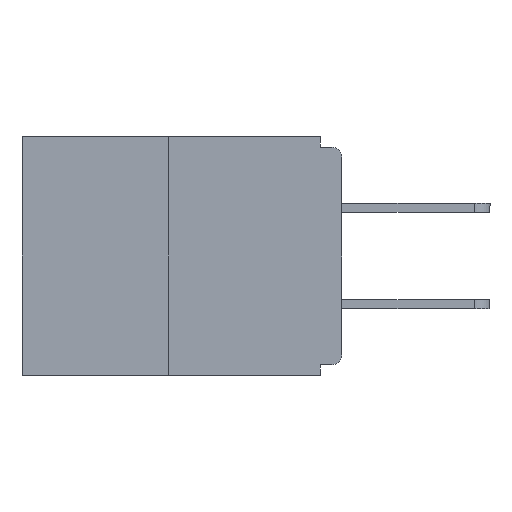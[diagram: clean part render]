
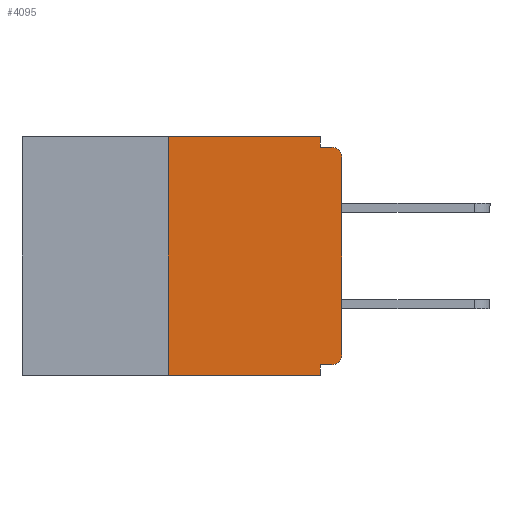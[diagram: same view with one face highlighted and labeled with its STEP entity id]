
A CAD part, left-side view. The second image highlights one B-rep face of the part: STEP entity #4095.
In plain terms, the highlighted planar face has unit normal (-1, 0, 0).
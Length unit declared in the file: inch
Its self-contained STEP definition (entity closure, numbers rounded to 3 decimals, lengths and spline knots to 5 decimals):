
#136 = EDGE_CURVE ( 'NONE', #3939, #10348, #20464, .T. ) ;
#175 = VECTOR ( 'NONE', #2229, 39.37008 ) ;
#220 = CARTESIAN_POINT ( 'NONE',  ( 0., 0.46, 0. ) ) ;
#252 = ORIENTED_EDGE ( 'NONE', *, *, #10432, .F. ) ;
#340 = CARTESIAN_POINT ( 'NONE',  ( 0., 0., -0.03 ) ) ;
#493 = LINE ( 'NONE', #2127, #12126 ) ;
#1427 = VERTEX_POINT ( 'NONE', #12064 ) ;
#2127 = CARTESIAN_POINT ( 'NONE',  ( 0., 0.46, -0.343 ) ) ;
#2229 = DIRECTION ( 'NONE',  ( 0., -1., 0. ) ) ;
#2239 = DIRECTION ( 'NONE',  ( 0., 0., -1. ) ) ;
#2779 = LINE ( 'NONE', #7794, #8220 ) ;
#2801 = CARTESIAN_POINT ( 'NONE',  ( 0., 0.015, -0.015 ) ) ;
#2879 = ORIENTED_EDGE ( 'NONE', *, *, #3324, .F. ) ;
#3036 = EDGE_CURVE ( 'NONE', #13021, #10348, #493, .T. ) ;
#3054 = ORIENTED_EDGE ( 'NONE', *, *, #16053, .F. ) ;
#3324 = EDGE_CURVE ( 'NONE', #13021, #15817, #4747, .T. ) ;
#3610 = CARTESIAN_POINT ( 'NONE',  ( 0., 0.015, -0.328 ) ) ;
#3939 = VERTEX_POINT ( 'NONE', #9247 ) ;
#4095 = ADVANCED_FACE ( 'NONE', ( #6446 ), #19255, .F. ) ;
#4668 = CARTESIAN_POINT ( 'NONE',  ( 0., 0., -0.328 ) ) ;
#4747 = LINE ( 'NONE', #15003, #13897 ) ;
#4929 = CARTESIAN_POINT ( 'NONE',  ( 0., 0.031, 0. ) ) ;
#5041 = CIRCLE ( 'NONE', #9271, 0.015 ) ;
#5063 = LINE ( 'NONE', #4668, #12690 ) ;
#5141 = DIRECTION ( 'NONE',  ( 0., -1., 0. ) ) ;
#5260 = VERTEX_POINT ( 'NONE', #340 ) ;
#5685 = LINE ( 'NONE', #8404, #175 ) ;
#5875 = ORIENTED_EDGE ( 'NONE', *, *, #16326, .T. ) ;
#6446 = FACE_OUTER_BOUND ( 'NONE', #13873, .T. ) ;
#6505 = DIRECTION ( 'NONE',  ( 1., 0., 0. ) ) ;
#6519 = DIRECTION ( 'NONE',  ( 0., 0., -1. ) ) ;
#6920 = ORIENTED_EDGE ( 'NONE', *, *, #15191, .F. ) ;
#7124 = ORIENTED_EDGE ( 'NONE', *, *, #12828, .F. ) ;
#7405 = CARTESIAN_POINT ( 'NONE',  ( 0., 0.46, 0. ) ) ;
#7550 = CARTESIAN_POINT ( 'NONE',  ( 0., 0.031, -0.015 ) ) ;
#7794 = CARTESIAN_POINT ( 'NONE',  ( 0., 0., 0. ) ) ;
#8066 = VERTEX_POINT ( 'NONE', #2801 ) ;
#8220 = VECTOR ( 'NONE', #15786, 39.37008 ) ;
#8404 = CARTESIAN_POINT ( 'NONE',  ( 0., 0., -0.015 ) ) ;
#8545 = VECTOR ( 'NONE', #20500, 39.37008 ) ;
#8614 = DIRECTION ( 'NONE',  ( -1., 0., 0. ) ) ;
#8753 = LINE ( 'NONE', #4929, #11954 ) ;
#8851 = CIRCLE ( 'NONE', #18661, 0.015 ) ;
#9132 = VERTEX_POINT ( 'NONE', #15244 ) ;
#9247 = CARTESIAN_POINT ( 'NONE',  ( 0., 0.031, -0.328 ) ) ;
#9271 = AXIS2_PLACEMENT_3D ( 'NONE', #16479, #8614, #2239 ) ;
#9798 = VERTEX_POINT ( 'NONE', #7550 ) ;
#9909 = DIRECTION ( 'NONE',  ( 0., 0., -1. ) ) ;
#10045 = DIRECTION ( 'NONE',  ( -1., 0., 0. ) ) ;
#10348 = VERTEX_POINT ( 'NONE', #18859 ) ;
#10432 = EDGE_CURVE ( 'NONE', #9132, #9798, #8753, .T. ) ;
#10541 = LINE ( 'NONE', #7405, #11522 ) ;
#11482 = CARTESIAN_POINT ( 'NONE',  ( 0., 0.015, -0.03 ) ) ;
#11522 = VECTOR ( 'NONE', #13494, 39.37008 ) ;
#11954 = VECTOR ( 'NONE', #6519, 39.37008 ) ;
#12064 = CARTESIAN_POINT ( 'NONE',  ( 0., 0., -0.313 ) ) ;
#12126 = VECTOR ( 'NONE', #5141, 39.37008 ) ;
#12532 = DIRECTION ( 'NONE',  ( 0., 1., 0. ) ) ;
#12570 = CARTESIAN_POINT ( 'NONE',  ( 0., 0.031, -0.343 ) ) ;
#12571 = ORIENTED_EDGE ( 'NONE', *, *, #3036, .T. ) ;
#12690 = VECTOR ( 'NONE', #12532, 39.37008 ) ;
#12828 = EDGE_CURVE ( 'NONE', #9798, #8066, #5685, .T. ) ;
#13021 = VERTEX_POINT ( 'NONE', #13996 ) ;
#13199 = AXIS2_PLACEMENT_3D ( 'NONE', #220, #6505, #17506 ) ;
#13381 = EDGE_CURVE ( 'NONE', #5260, #8066, #8851, .T. ) ;
#13494 = DIRECTION ( 'NONE',  ( 0., -1., 0. ) ) ;
#13598 = DIRECTION ( 'NONE',  ( 0., 0., 1. ) ) ;
#13873 = EDGE_LOOP ( 'NONE', ( #6920, #2879, #12571, #15450, #3054, #17850, #5875, #15008, #7124, #252 ) ) ;
#13897 = VECTOR ( 'NONE', #13598, 39.37008 ) ;
#13996 = CARTESIAN_POINT ( 'NONE',  ( 0., 0.25, -0.343 ) ) ;
#15003 = CARTESIAN_POINT ( 'NONE',  ( 0., 0.25, 0. ) ) ;
#15008 = ORIENTED_EDGE ( 'NONE', *, *, #13381, .T. ) ;
#15191 = EDGE_CURVE ( 'NONE', #15817, #9132, #10541, .T. ) ;
#15244 = CARTESIAN_POINT ( 'NONE',  ( 0., 0.031, 0. ) ) ;
#15450 = ORIENTED_EDGE ( 'NONE', *, *, #136, .F. ) ;
#15786 = DIRECTION ( 'NONE',  ( 0., 0., 1. ) ) ;
#15817 = VERTEX_POINT ( 'NONE', #17685 ) ;
#16053 = EDGE_CURVE ( 'NONE', #20052, #3939, #5063, .T. ) ;
#16326 = EDGE_CURVE ( 'NONE', #1427, #5260, #2779, .T. ) ;
#16479 = CARTESIAN_POINT ( 'NONE',  ( 0., 0.015, -0.313 ) ) ;
#16612 = EDGE_CURVE ( 'NONE', #20052, #1427, #5041, .T. ) ;
#17506 = DIRECTION ( 'NONE',  ( 0., 0., -1. ) ) ;
#17685 = CARTESIAN_POINT ( 'NONE',  ( 0., 0.25, 0. ) ) ;
#17850 = ORIENTED_EDGE ( 'NONE', *, *, #16612, .T. ) ;
#18661 = AXIS2_PLACEMENT_3D ( 'NONE', #11482, #10045, #9909 ) ;
#18859 = CARTESIAN_POINT ( 'NONE',  ( 0., 0.031, -0.343 ) ) ;
#19255 = PLANE ( 'NONE',  #13199 ) ;
#20052 = VERTEX_POINT ( 'NONE', #3610 ) ;
#20464 = LINE ( 'NONE', #12570, #8545 ) ;
#20500 = DIRECTION ( 'NONE',  ( 0., 0., -1. ) ) ;
